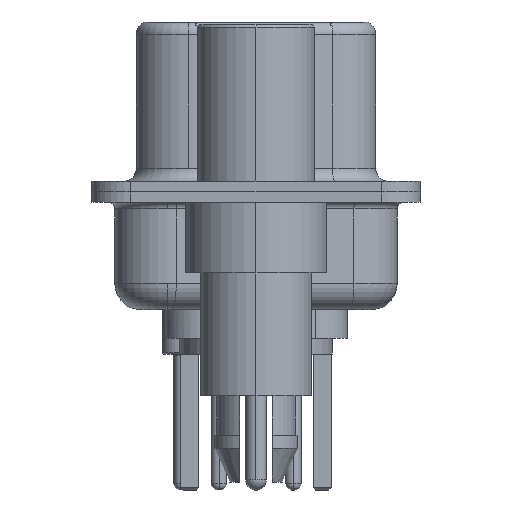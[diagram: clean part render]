
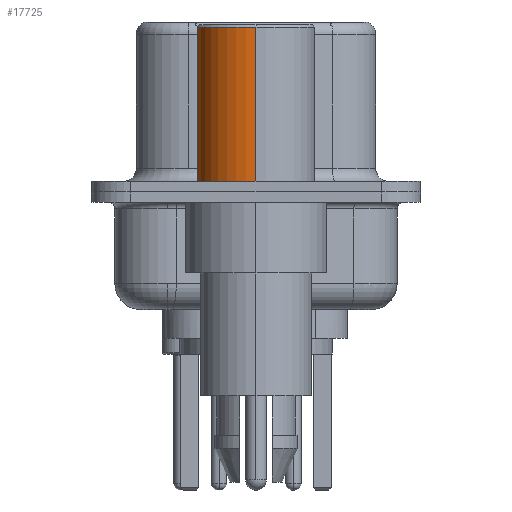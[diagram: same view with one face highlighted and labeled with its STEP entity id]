
A CAD part, left-side view. The second image highlights one B-rep face of the part: STEP entity #17725.
In plain terms, the highlighted cylindrical face has radius 2.25 mm (diameter 4.5 mm), a partial arc.
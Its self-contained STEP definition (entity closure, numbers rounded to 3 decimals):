
#1141 = CARTESIAN_POINT ( 'NONE',  ( 0., 0., 0.4 ) ) ;
#2630 = CARTESIAN_POINT ( 'NONE',  ( 2.25, 0., 0.4 ) ) ;
#3210 = DIRECTION ( 'NONE',  ( 1., 0., 0. ) ) ;
#3702 = VERTEX_POINT ( 'NONE', #2630 ) ;
#5241 = DIRECTION ( 'NONE',  ( 0., 0., 1. ) ) ;
#5303 = CARTESIAN_POINT ( 'NONE',  ( -2.25, 0., 0.581 ) ) ;
#5358 = CARTESIAN_POINT ( 'NONE',  ( 0., 0., 6.3 ) ) ;
#6980 = VECTOR ( 'NONE', #17539, 1000. ) ;
#7163 = EDGE_CURVE ( 'NONE', #16088, #13415, #21995, .T. ) ;
#7245 = CARTESIAN_POINT ( 'NONE',  ( 2.25, 0., 0.581 ) ) ;
#7247 = ORIENTED_EDGE ( 'NONE', *, *, #14974, .F. ) ;
#7360 = DIRECTION ( 'NONE',  ( 1., 0., 0. ) ) ;
#7488 = CARTESIAN_POINT ( 'NONE',  ( -2.25, 0., 6.3 ) ) ;
#8048 = CARTESIAN_POINT ( 'NONE',  ( 2.25, 0., 6.3 ) ) ;
#11209 = DIRECTION ( 'NONE',  ( 1., 0., 0. ) ) ;
#13415 = VERTEX_POINT ( 'NONE', #7488 ) ;
#13602 = ORIENTED_EDGE ( 'NONE', *, *, #17702, .T. ) ;
#13703 = FACE_OUTER_BOUND ( 'NONE', #22901, .T. ) ;
#14974 = EDGE_CURVE ( 'NONE', #3702, #22077, #16373, .T. ) ;
#15275 = CIRCLE ( 'NONE', #19148, 2.25 ) ;
#15382 = DIRECTION ( 'NONE',  ( 0., 0., 1. ) ) ;
#15431 = ORIENTED_EDGE ( 'NONE', *, *, #18442, .F. ) ;
#16088 = VERTEX_POINT ( 'NONE', #19328 ) ;
#16373 = LINE ( 'NONE', #7245, #22417 ) ;
#16511 = AXIS2_PLACEMENT_3D ( 'NONE', #1141, #15382, #3210 ) ;
#17481 = CARTESIAN_POINT ( 'NONE',  ( 0., 0., 0.581 ) ) ;
#17539 = DIRECTION ( 'NONE',  ( 0., 0., 1. ) ) ;
#17702 = EDGE_CURVE ( 'NONE', #3702, #16088, #25291, .T. ) ;
#17725 = ADVANCED_FACE ( 'NONE', ( #13703 ), #23993, .T. ) ;
#18353 = ORIENTED_EDGE ( 'NONE', *, *, #7163, .T. ) ;
#18442 = EDGE_CURVE ( 'NONE', #22077, #13415, #15275, .T. ) ;
#19148 = AXIS2_PLACEMENT_3D ( 'NONE', #5358, #19668, #7360 ) ;
#19328 = CARTESIAN_POINT ( 'NONE',  ( -2.25, 0., 0.4 ) ) ;
#19668 = DIRECTION ( 'NONE',  ( 0., 0., 1. ) ) ;
#21543 = DIRECTION ( 'NONE',  ( 0., 0., 1. ) ) ;
#21965 = AXIS2_PLACEMENT_3D ( 'NONE', #17481, #5241, #11209 ) ;
#21995 = LINE ( 'NONE', #5303, #6980 ) ;
#22077 = VERTEX_POINT ( 'NONE', #8048 ) ;
#22417 = VECTOR ( 'NONE', #21543, 1000. ) ;
#22901 = EDGE_LOOP ( 'NONE', ( #13602, #18353, #15431, #7247 ) ) ;
#23993 = CYLINDRICAL_SURFACE ( 'NONE', #21965, 2.25 ) ;
#25291 = CIRCLE ( 'NONE', #16511, 2.25 ) ;
